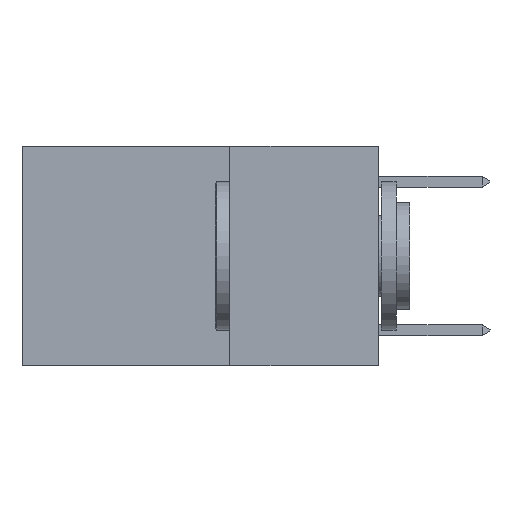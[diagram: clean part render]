
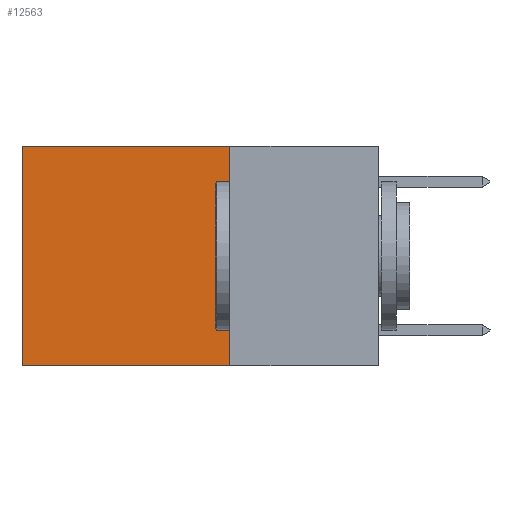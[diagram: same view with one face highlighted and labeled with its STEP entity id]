
A CAD part, left-side view. The second image highlights one B-rep face of the part: STEP entity #12563.
In plain terms, the highlighted planar face has unit normal (-1, 0, 0).
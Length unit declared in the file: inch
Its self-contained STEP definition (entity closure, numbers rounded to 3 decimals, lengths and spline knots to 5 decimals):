
#780 = ORIENTED_EDGE ( 'NONE', *, *, #8324, .T. ) ;
#1520 = VERTEX_POINT ( 'NONE', #12896 ) ;
#1552 = CARTESIAN_POINT ( 'NONE',  ( 0.2625, 0.25, 0. ) ) ;
#2029 = DIRECTION ( 'NONE',  ( 0., 0., -1. ) ) ;
#2064 = CARTESIAN_POINT ( 'NONE',  ( 0.2625, 0.25, 0. ) ) ;
#2428 = DIRECTION ( 'NONE',  ( 0., 1., 0. ) ) ;
#2544 = LINE ( 'NONE', #15394, #2566 ) ;
#2566 = VECTOR ( 'NONE', #15354, 39.37008 ) ;
#2701 = FACE_OUTER_BOUND ( 'NONE', #15001, .T. ) ;
#3062 = VERTEX_POINT ( 'NONE', #15189 ) ;
#4050 = EDGE_CURVE ( 'NONE', #4804, #9238, #2544, .T. ) ;
#4804 = VERTEX_POINT ( 'NONE', #11680 ) ;
#5314 = EDGE_CURVE ( 'NONE', #1520, #4804, #20274, .T. ) ;
#6884 = PLANE ( 'NONE',  #19992 ) ;
#8324 = EDGE_CURVE ( 'NONE', #3062, #9238, #18480, .T. ) ;
#8540 = DIRECTION ( 'NONE',  ( 0., 0., -1. ) ) ;
#9238 = VERTEX_POINT ( 'NONE', #11018 ) ;
#10762 = DIRECTION ( 'NONE',  ( 0., 0., -1. ) ) ;
#10970 = CARTESIAN_POINT ( 'NONE',  ( 0.2625, 0.6, 0. ) ) ;
#11018 = CARTESIAN_POINT ( 'NONE',  ( 0.2625, 0.6, -0.37 ) ) ;
#11680 = CARTESIAN_POINT ( 'NONE',  ( 0.2625, 0.25, -0.37 ) ) ;
#12563 = ADVANCED_FACE ( 'NONE', ( #2701 ), #6884, .F. ) ;
#12839 = EDGE_CURVE ( 'NONE', #1520, #3062, #20082, .T. ) ;
#12877 = ORIENTED_EDGE ( 'NONE', *, *, #4050, .F. ) ;
#12896 = CARTESIAN_POINT ( 'NONE',  ( 0.2625, 0.25, 0. ) ) ;
#13981 = CARTESIAN_POINT ( 'NONE',  ( 0.2625, 0.25, 0. ) ) ;
#15001 = EDGE_LOOP ( 'NONE', ( #780, #12877, #17930, #19851 ) ) ;
#15189 = CARTESIAN_POINT ( 'NONE',  ( 0.2625, 0.6, 0. ) ) ;
#15354 = DIRECTION ( 'NONE',  ( 0., 1., 0. ) ) ;
#15394 = CARTESIAN_POINT ( 'NONE',  ( 0.2625, 0.25, -0.37 ) ) ;
#17930 = ORIENTED_EDGE ( 'NONE', *, *, #5314, .F. ) ;
#17946 = DIRECTION ( 'NONE',  ( 1., 0., 0. ) ) ;
#18461 = VECTOR ( 'NONE', #2029, 39.37008 ) ;
#18480 = LINE ( 'NONE', #10970, #19057 ) ;
#19057 = VECTOR ( 'NONE', #10762, 39.37008 ) ;
#19268 = VECTOR ( 'NONE', #2428, 39.37008 ) ;
#19851 = ORIENTED_EDGE ( 'NONE', *, *, #12839, .T. ) ;
#19992 = AXIS2_PLACEMENT_3D ( 'NONE', #1552, #17946, #8540 ) ;
#20082 = LINE ( 'NONE', #13981, #19268 ) ;
#20274 = LINE ( 'NONE', #2064, #18461 ) ;
